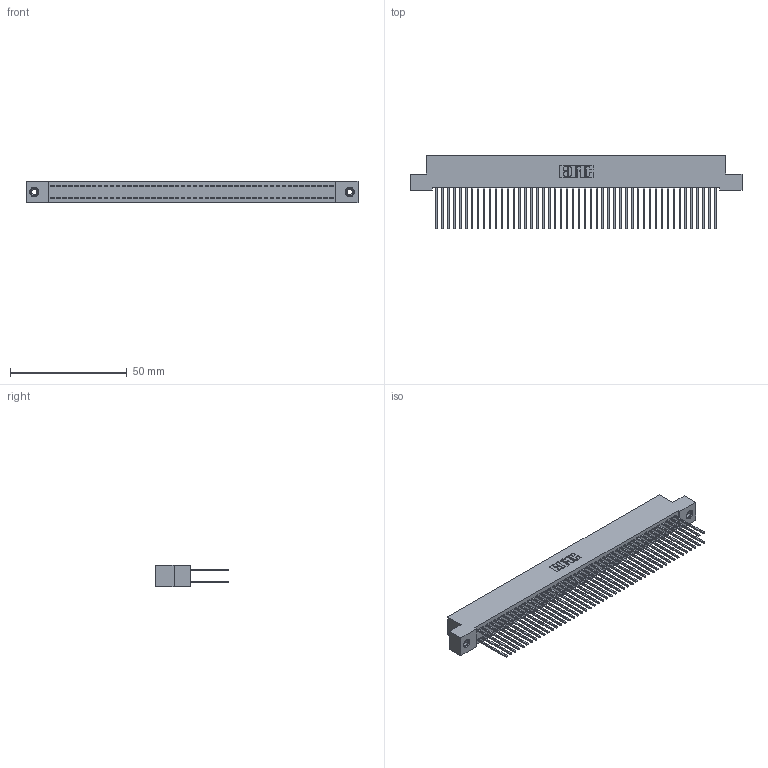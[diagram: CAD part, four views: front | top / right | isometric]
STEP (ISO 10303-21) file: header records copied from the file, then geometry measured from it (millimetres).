
FILE_DESCRIPTION (( 'STEP AP203' ), '1' );
FILE_NAME ('342-096-542-208.STEP', '2018-08-14T03:15:22', ( '' ), ( '' ), 'SwSTEP 2.0', 'SolidWorks 2016', '' );
FILE_SCHEMA (( 'CONFIG_CONTROL_DESIGN' ));
Length unit declared in the file: inch
Products named in the file (4): 345-292-001_345-293-142; 345-250-001_345-250-003-102; 342-096-542-208; 342 Part_TI
Assembly tree (99 placements, depth 2):
  342-096-542-208
    342 Part_TI
    345-292-001_345-293-142  x96
    345-250-001_345-250-003-102  x2
Bounding box: 142.24 x 31.63 x 9.4 mm (x, y, z)
Volume: 13250.5 mm3; surface area: 23734.9 mm2
Topology: 99 solids, 99 shells, 5162 faces, 15315 edges, 10074 vertices
Faces by surface type: plane 3554, cylinder 1592, cone 12, torus 4
Entity records: 31176 total; most frequent: CARTESIAN_POINT 5141, ORIENTED_EDGE 5070, DIRECTION 4413, EDGE_CURVE 2535, LINE 2387, VECTOR 2387, VERTEX_POINT 1684, AXIS2_PLACEMENT_3D 1013
